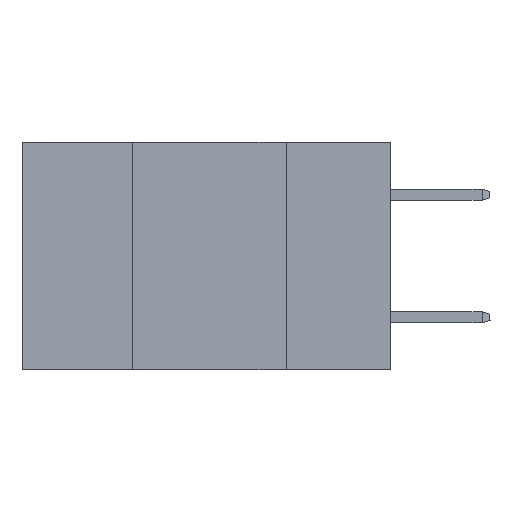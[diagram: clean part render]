
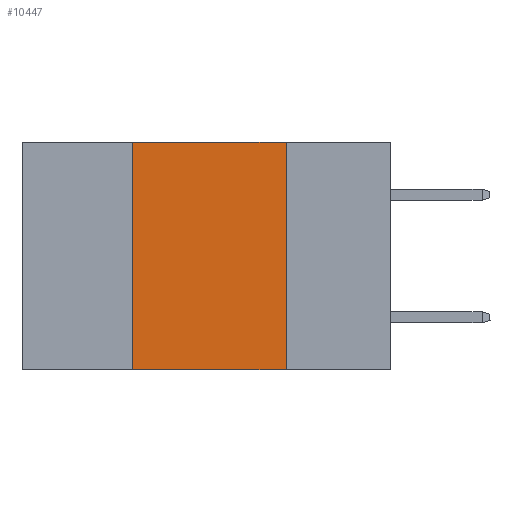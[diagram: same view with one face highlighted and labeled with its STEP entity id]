
A CAD part, left-side view. The second image highlights one B-rep face of the part: STEP entity #10447.
In plain terms, the highlighted planar face has unit normal (-1, 0, 0).
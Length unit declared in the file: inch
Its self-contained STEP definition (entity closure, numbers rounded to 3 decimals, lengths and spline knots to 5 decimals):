
#191 = LINE ( 'NONE', #13334, #3049 ) ;
#2178 = FACE_OUTER_BOUND ( 'NONE', #19534, .T. ) ;
#2327 = EDGE_CURVE ( 'NONE', #20995, #28271, #43160, .T. ) ;
#3049 = VECTOR ( 'NONE', #36732, 39.37008 ) ;
#3384 = ORIENTED_EDGE ( 'NONE', *, *, #2327, .F. ) ;
#3743 = LINE ( 'NONE', #13761, #20108 ) ;
#5285 = PLANE ( 'NONE',  #23726 ) ;
#5295 = CARTESIAN_POINT ( 'NONE',  ( 0., 0.6, 0. ) ) ;
#7064 = DIRECTION ( 'NONE',  ( 0., 0., 1. ) ) ;
#9991 = CARTESIAN_POINT ( 'NONE',  ( 0., 0.42, -0.37 ) ) ;
#10016 = ORIENTED_EDGE ( 'NONE', *, *, #27391, .F. ) ;
#10447 = ADVANCED_FACE ( 'NONE', ( #2178 ), #5285, .F. ) ;
#12193 = DIRECTION ( 'NONE',  ( 1., 0., 0. ) ) ;
#13334 = CARTESIAN_POINT ( 'NONE',  ( 0., 0.6, -0.37 ) ) ;
#13761 = CARTESIAN_POINT ( 'NONE',  ( 0., 0.42, 0. ) ) ;
#13961 = EDGE_CURVE ( 'NONE', #28271, #22021, #39441, .T. ) ;
#14934 = CARTESIAN_POINT ( 'NONE',  ( 0., 0.17, 0. ) ) ;
#18275 = VERTEX_POINT ( 'NONE', #9991 ) ;
#18859 = DIRECTION ( 'NONE',  ( 0., 0., -1. ) ) ;
#19534 = EDGE_LOOP ( 'NONE', ( #34405, #3384, #10016, #33144 ) ) ;
#20108 = VECTOR ( 'NONE', #7064, 39.37008 ) ;
#20995 = VERTEX_POINT ( 'NONE', #30779 ) ;
#22021 = VERTEX_POINT ( 'NONE', #36728 ) ;
#22869 = CARTESIAN_POINT ( 'NONE',  ( 0., 0.6, 0. ) ) ;
#23726 = AXIS2_PLACEMENT_3D ( 'NONE', #22869, #12193, #18859 ) ;
#24255 = VECTOR ( 'NONE', #28519, 39.37008 ) ;
#27391 = EDGE_CURVE ( 'NONE', #18275, #20995, #3743, .T. ) ;
#27685 = CARTESIAN_POINT ( 'NONE',  ( 0., 0.17, 0. ) ) ;
#28271 = VERTEX_POINT ( 'NONE', #27685 ) ;
#28519 = DIRECTION ( 'NONE',  ( 0., 0., -1. ) ) ;
#29148 = EDGE_CURVE ( 'NONE', #18275, #22021, #191, .T. ) ;
#30779 = CARTESIAN_POINT ( 'NONE',  ( 0., 0.42, 0. ) ) ;
#32467 = DIRECTION ( 'NONE',  ( 0., -1., 0. ) ) ;
#33144 = ORIENTED_EDGE ( 'NONE', *, *, #29148, .T. ) ;
#34405 = ORIENTED_EDGE ( 'NONE', *, *, #13961, .F. ) ;
#36728 = CARTESIAN_POINT ( 'NONE',  ( 0., 0.17, -0.37 ) ) ;
#36732 = DIRECTION ( 'NONE',  ( 0., -1., 0. ) ) ;
#39441 = LINE ( 'NONE', #14934, #24255 ) ;
#43160 = LINE ( 'NONE', #5295, #43800 ) ;
#43800 = VECTOR ( 'NONE', #32467, 39.37008 ) ;
